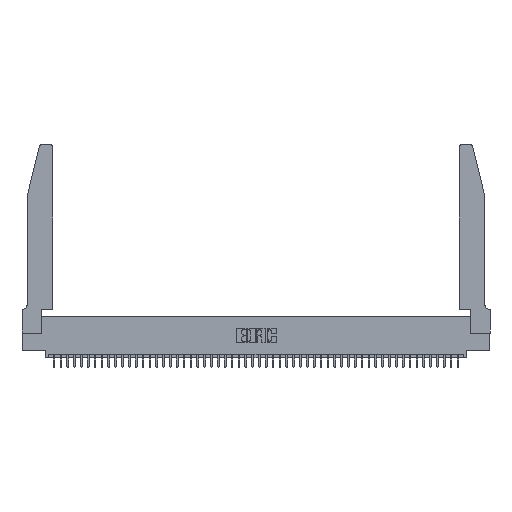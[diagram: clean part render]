
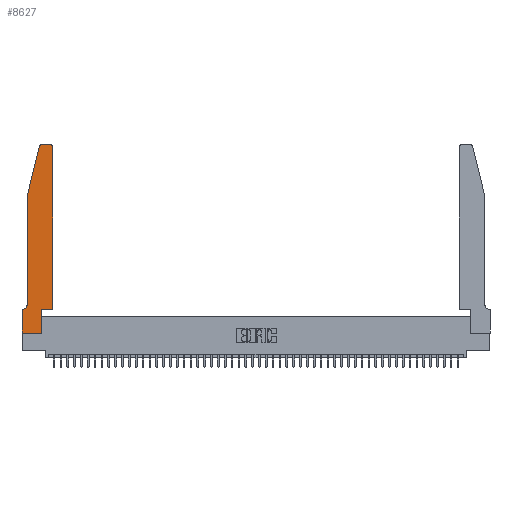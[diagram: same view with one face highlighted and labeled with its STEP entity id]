
A CAD part, top view. The second image highlights one B-rep face of the part: STEP entity #8627.
In plain terms, the highlighted planar face has unit normal (0, 0, 1).
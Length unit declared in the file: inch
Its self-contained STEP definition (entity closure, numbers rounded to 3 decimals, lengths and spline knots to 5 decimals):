
#185 = CARTESIAN_POINT ( 'NONE',  ( 0.4505, 0.35, 0.37 ) ) ;
#270 = VECTOR ( 'NONE', #18716, 39.37008 ) ;
#1254 = LINE ( 'NONE', #28023, #19476 ) ;
#1485 = EDGE_CURVE ( 'NONE', #42792, #37860, #1254, .T. ) ;
#2809 = EDGE_CURVE ( 'NONE', #41928, #7357, #22952, .T. ) ;
#3912 = EDGE_CURVE ( 'NONE', #37860, #36373, #5257, .T. ) ;
#4003 = EDGE_CURVE ( 'NONE', #6689, #11935, #11994, .T. ) ;
#4036 = CARTESIAN_POINT ( 'NONE',  ( 0., 0., 0.37 ) ) ;
#4154 = EDGE_CURVE ( 'NONE', #11935, #42792, #49435, .T. ) ;
#4887 = DIRECTION ( 'NONE',  ( 0., 1., 0. ) ) ;
#5257 = LINE ( 'NONE', #185, #44724 ) ;
#5582 = EDGE_CURVE ( 'NONE', #8161, #16158, #39832, .T. ) ;
#5597 = DIRECTION ( 'NONE',  ( 1., 0., 0. ) ) ;
#5668 = DIRECTION ( 'NONE',  ( 0., 0., -1. ) ) ;
#6689 = VERTEX_POINT ( 'NONE', #49322 ) ;
#7302 = VECTOR ( 'NONE', #17791, 39.37008 ) ;
#7357 = VERTEX_POINT ( 'NONE', #37941 ) ;
#8161 = VERTEX_POINT ( 'NONE', #42864 ) ;
#8627 = ADVANCED_FACE ( 'NONE', ( #14638 ), #19141, .T. ) ;
#9689 = CIRCLE ( 'NONE', #44082, 0.03 ) ;
#10583 = CARTESIAN_POINT ( 'NONE',  ( 0.284, 2.72, 0.37 ) ) ;
#10632 = AXIS2_PLACEMENT_3D ( 'NONE', #34258, #45664, #23011 ) ;
#10929 = DIRECTION ( 'NONE',  ( 0., 0., 1. ) ) ;
#11935 = VERTEX_POINT ( 'NONE', #4036 ) ;
#11994 = LINE ( 'NONE', #16350, #31175 ) ;
#13166 = EDGE_CURVE ( 'NONE', #43439, #8161, #9689, .T. ) ;
#14099 = DIRECTION ( 'NONE',  ( 0., 1., 0. ) ) ;
#14119 = DIRECTION ( 'NONE',  ( -0.239, -0.971, 0. ) ) ;
#14513 = DIRECTION ( 'NONE',  ( 1., 0., 0. ) ) ;
#14572 = EDGE_CURVE ( 'NONE', #34754, #6689, #39446, .T. ) ;
#14638 = FACE_OUTER_BOUND ( 'NONE', #36343, .T. ) ;
#14875 = ORIENTED_EDGE ( 'NONE', *, *, #35142, .T. ) ;
#15702 = AXIS2_PLACEMENT_3D ( 'NONE', #10583, #37236, #14513 ) ;
#16158 = VERTEX_POINT ( 'NONE', #35279 ) ;
#16350 = CARTESIAN_POINT ( 'NONE',  ( 0., 0., 0.37 ) ) ;
#16486 = ORIENTED_EDGE ( 'NONE', *, *, #4154, .T. ) ;
#17133 = ORIENTED_EDGE ( 'NONE', *, *, #2809, .T. ) ;
#17791 = DIRECTION ( 'NONE',  ( 0., -1., 0. ) ) ;
#17926 = CARTESIAN_POINT ( 'NONE',  ( 0.4505, 0.35, 0.37 ) ) ;
#17948 = CARTESIAN_POINT ( 'NONE',  ( 0.25487, 2.72718, 0.37 ) ) ;
#18378 = ORIENTED_EDGE ( 'NONE', *, *, #1485, .T. ) ;
#18716 = DIRECTION ( 'NONE',  ( -1., 0., 0. ) ) ;
#19141 = PLANE ( 'NONE',  #10632 ) ;
#19300 = VECTOR ( 'NONE', #45765, 39.37008 ) ;
#19476 = VECTOR ( 'NONE', #4887, 39.37008 ) ;
#19496 = CARTESIAN_POINT ( 'NONE',  ( 0.0055, 0.35, 0.37 ) ) ;
#19533 = ORIENTED_EDGE ( 'NONE', *, *, #13166, .T. ) ;
#20269 = EDGE_CURVE ( 'NONE', #16158, #41928, #28790, .T. ) ;
#20746 = VECTOR ( 'NONE', #14099, 39.37008 ) ;
#21198 = ORIENTED_EDGE ( 'NONE', *, *, #14572, .T. ) ;
#21744 = VECTOR ( 'NONE', #14119, 39.37008 ) ;
#22064 = CIRCLE ( 'NONE', #25212, 0.07 ) ;
#22194 = ORIENTED_EDGE ( 'NONE', *, *, #5582, .T. ) ;
#22952 = LINE ( 'NONE', #29323, #21744 ) ;
#23011 = DIRECTION ( 'NONE',  ( 1., 0., 0. ) ) ;
#23044 = ORIENTED_EDGE ( 'NONE', *, *, #20269, .T. ) ;
#24717 = EDGE_CURVE ( 'NONE', #36373, #43439, #40848, .T. ) ;
#25187 = ORIENTED_EDGE ( 'NONE', *, *, #24717, .T. ) ;
#25212 = AXIS2_PLACEMENT_3D ( 'NONE', #28775, #5668, #32572 ) ;
#25337 = VERTEX_POINT ( 'NONE', #26095 ) ;
#26095 = CARTESIAN_POINT ( 'NONE',  ( 0.0755, 0.42, 0.37 ) ) ;
#26750 = CARTESIAN_POINT ( 'NONE',  ( 0.2865, 0., 0.37 ) ) ;
#28023 = CARTESIAN_POINT ( 'NONE',  ( 0.2865, 0.35, 0.37 ) ) ;
#28597 = ORIENTED_EDGE ( 'NONE', *, *, #3912, .T. ) ;
#28775 = CARTESIAN_POINT ( 'NONE',  ( 0.0055, 0.42, 0.37 ) ) ;
#28790 = CIRCLE ( 'NONE', #15702, 0.03 ) ;
#29323 = CARTESIAN_POINT ( 'NONE',  ( 0.0755, 2., 0.37 ) ) ;
#31175 = VECTOR ( 'NONE', #35287, 39.37008 ) ;
#31656 = CARTESIAN_POINT ( 'NONE',  ( 0.4505, 2.72, 0.37 ) ) ;
#32297 = ORIENTED_EDGE ( 'NONE', *, *, #4003, .T. ) ;
#32571 = EDGE_CURVE ( 'NONE', #25337, #34754, #22064, .T. ) ;
#32572 = DIRECTION ( 'NONE',  ( -1., 0., 0. ) ) ;
#33817 = CARTESIAN_POINT ( 'NONE',  ( 0.4205, 2.72, 0.37 ) ) ;
#34258 = CARTESIAN_POINT ( 'NONE',  ( 0., 0.35, 0.37 ) ) ;
#34754 = VERTEX_POINT ( 'NONE', #19496 ) ;
#35142 = EDGE_CURVE ( 'NONE', #7357, #25337, #45522, .T. ) ;
#35279 = CARTESIAN_POINT ( 'NONE',  ( 0.284, 2.75, 0.37 ) ) ;
#35287 = DIRECTION ( 'NONE',  ( 0., -1., 0. ) ) ;
#36254 = CARTESIAN_POINT ( 'NONE',  ( 0., 0., 0.37 ) ) ;
#36343 = EDGE_LOOP ( 'NONE', ( #22194, #23044, #17133, #14875, #40674, #21198, #32297, #16486, #18378, #28597, #25187, #19533 ) ) ;
#36373 = VERTEX_POINT ( 'NONE', #47833 ) ;
#36688 = CARTESIAN_POINT ( 'NONE',  ( 0.0755, 2., 0.37 ) ) ;
#37236 = DIRECTION ( 'NONE',  ( 0., 0., 1. ) ) ;
#37556 = DIRECTION ( 'NONE',  ( 1., 0., 0. ) ) ;
#37860 = VERTEX_POINT ( 'NONE', #45532 ) ;
#37941 = CARTESIAN_POINT ( 'NONE',  ( 0.0755, 2., 0.37 ) ) ;
#38564 = DIRECTION ( 'NONE',  ( 1., 0., 0. ) ) ;
#39446 = LINE ( 'NONE', #41926, #19300 ) ;
#39832 = LINE ( 'NONE', #41396, #270 ) ;
#40674 = ORIENTED_EDGE ( 'NONE', *, *, #32571, .T. ) ;
#40848 = LINE ( 'NONE', #17926, #20746 ) ;
#41396 = CARTESIAN_POINT ( 'NONE',  ( 0.2605, 2.75, 0.37 ) ) ;
#41926 = CARTESIAN_POINT ( 'NONE',  ( 0.0755, 0.35, 0.37 ) ) ;
#41928 = VERTEX_POINT ( 'NONE', #17948 ) ;
#42792 = VERTEX_POINT ( 'NONE', #26750 ) ;
#42864 = CARTESIAN_POINT ( 'NONE',  ( 0.4205, 2.75, 0.37 ) ) ;
#43439 = VERTEX_POINT ( 'NONE', #31656 ) ;
#44082 = AXIS2_PLACEMENT_3D ( 'NONE', #33817, #10929, #37556 ) ;
#44724 = VECTOR ( 'NONE', #38564, 39.37008 ) ;
#45522 = LINE ( 'NONE', #36688, #7302 ) ;
#45532 = CARTESIAN_POINT ( 'NONE',  ( 0.2865, 0.35, 0.37 ) ) ;
#45664 = DIRECTION ( 'NONE',  ( 0., 0., 1. ) ) ;
#45765 = DIRECTION ( 'NONE',  ( -1., 0., 0. ) ) ;
#47833 = CARTESIAN_POINT ( 'NONE',  ( 0.4505, 0.35, 0.37 ) ) ;
#48230 = VECTOR ( 'NONE', #5597, 39.37008 ) ;
#49322 = CARTESIAN_POINT ( 'NONE',  ( 0., 0.35, 0.37 ) ) ;
#49435 = LINE ( 'NONE', #36254, #48230 ) ;
